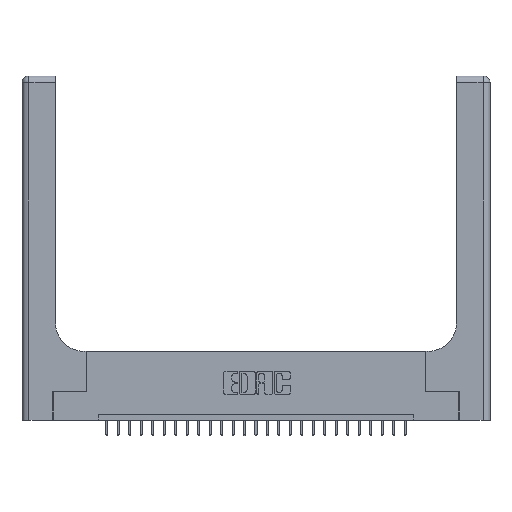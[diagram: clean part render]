
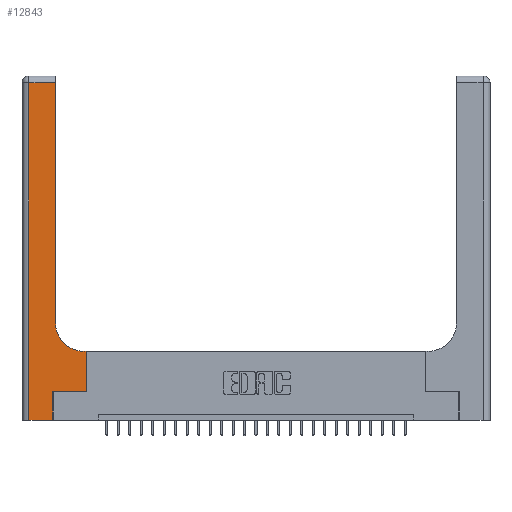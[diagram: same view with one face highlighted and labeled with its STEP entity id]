
A CAD part, top view. The second image highlights one B-rep face of the part: STEP entity #12843.
In plain terms, the highlighted planar face has unit normal (0, 0, 1).
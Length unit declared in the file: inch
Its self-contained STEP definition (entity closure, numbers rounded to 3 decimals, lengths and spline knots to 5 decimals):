
#403 = VERTEX_POINT ( 'NONE', #27520 ) ;
#743 = EDGE_LOOP ( 'NONE', ( #6027, #2777, #17085, #20887, #7346, #8097, #13744, #4555, #5136 ) ) ;
#778 = EDGE_CURVE ( 'NONE', #21902, #6032, #10229, .T. ) ;
#1618 = DIRECTION ( 'NONE',  ( 0., -1., 0. ) ) ;
#1889 = CARTESIAN_POINT ( 'NONE',  ( 0., 0., 0.37 ) ) ;
#2777 = ORIENTED_EDGE ( 'NONE', *, *, #16664, .T. ) ;
#3602 = CARTESIAN_POINT ( 'NONE',  ( 0.06, 2.94, 0.37 ) ) ;
#3624 = CARTESIAN_POINT ( 'NONE',  ( 0.269, 0., 0.37 ) ) ;
#4337 = DIRECTION ( 'NONE',  ( -1., 0., 0. ) ) ;
#4472 = CARTESIAN_POINT ( 'NONE',  ( 0.2915, 0.6, 0.37 ) ) ;
#4555 = ORIENTED_EDGE ( 'NONE', *, *, #15517, .T. ) ;
#5136 = ORIENTED_EDGE ( 'NONE', *, *, #16318, .T. ) ;
#5464 = DIRECTION ( 'NONE',  ( -1., 0., 0. ) ) ;
#5509 = LINE ( 'NONE', #5810, #17390 ) ;
#5621 = DIRECTION ( 'NONE',  ( -1., 0., 0. ) ) ;
#5810 = CARTESIAN_POINT ( 'NONE',  ( 0.06, 3., 0.37 ) ) ;
#6027 = ORIENTED_EDGE ( 'NONE', *, *, #16944, .T. ) ;
#6032 = VERTEX_POINT ( 'NONE', #25245 ) ;
#6249 = LINE ( 'NONE', #12702, #15602 ) ;
#6260 = EDGE_CURVE ( 'NONE', #12882, #21902, #9320, .T. ) ;
#6365 = DIRECTION ( 'NONE',  ( 1., 0., 0. ) ) ;
#6820 = LINE ( 'NONE', #4472, #7977 ) ;
#7346 = ORIENTED_EDGE ( 'NONE', *, *, #6260, .T. ) ;
#7562 = LINE ( 'NONE', #24616, #19625 ) ;
#7718 = CARTESIAN_POINT ( 'NONE',  ( 0., 3., 0.37 ) ) ;
#7977 = VECTOR ( 'NONE', #4337, 39.37008 ) ;
#8097 = ORIENTED_EDGE ( 'NONE', *, *, #778, .T. ) ;
#8233 = LINE ( 'NONE', #8536, #24083 ) ;
#8536 = CARTESIAN_POINT ( 'NONE',  ( 0.5585, 0.25, 0.37 ) ) ;
#9320 = LINE ( 'NONE', #19786, #27367 ) ;
#9348 = CIRCLE ( 'NONE', #10255, 0.25 ) ;
#9430 = FACE_OUTER_BOUND ( 'NONE', #743, .T. ) ;
#9842 = PLANE ( 'NONE',  #18192 ) ;
#10229 = LINE ( 'NONE', #16069, #27058 ) ;
#10255 = AXIS2_PLACEMENT_3D ( 'NONE', #17223, #19468, #25474 ) ;
#12702 = CARTESIAN_POINT ( 'NONE',  ( 0.2915, 3., 0.37 ) ) ;
#12843 = ADVANCED_FACE ( 'NONE', ( #9430 ), #9842, .F. ) ;
#12882 = VERTEX_POINT ( 'NONE', #3624 ) ;
#12930 = VERTEX_POINT ( 'NONE', #18705 ) ;
#13242 = VERTEX_POINT ( 'NONE', #24102 ) ;
#13744 = ORIENTED_EDGE ( 'NONE', *, *, #17756, .T. ) ;
#13872 = DIRECTION ( 'NONE',  ( 1., 0., 0. ) ) ;
#14234 = VERTEX_POINT ( 'NONE', #14402 ) ;
#14402 = CARTESIAN_POINT ( 'NONE',  ( 0.2915, 0.85, 0.37 ) ) ;
#15517 = EDGE_CURVE ( 'NONE', #403, #13242, #6820, .T. ) ;
#15602 = VECTOR ( 'NONE', #16732, 39.37008 ) ;
#16069 = CARTESIAN_POINT ( 'NONE',  ( 0.269, 0.25, 0.37 ) ) ;
#16318 = EDGE_CURVE ( 'NONE', #13242, #14234, #9348, .T. ) ;
#16664 = EDGE_CURVE ( 'NONE', #12930, #16796, #7562, .T. ) ;
#16732 = DIRECTION ( 'NONE',  ( 0., 1., 0. ) ) ;
#16796 = VERTEX_POINT ( 'NONE', #3602 ) ;
#16944 = EDGE_CURVE ( 'NONE', #14234, #12930, #6249, .T. ) ;
#17085 = ORIENTED_EDGE ( 'NONE', *, *, #23357, .T. ) ;
#17223 = CARTESIAN_POINT ( 'NONE',  ( 0.5415, 0.85, 0.37 ) ) ;
#17390 = VECTOR ( 'NONE', #1618, 39.37008 ) ;
#17756 = EDGE_CURVE ( 'NONE', #6032, #403, #8233, .T. ) ;
#18192 = AXIS2_PLACEMENT_3D ( 'NONE', #7718, #24766, #5621 ) ;
#18705 = CARTESIAN_POINT ( 'NONE',  ( 0.2915, 2.94, 0.37 ) ) ;
#19468 = DIRECTION ( 'NONE',  ( 0., 0., -1. ) ) ;
#19625 = VECTOR ( 'NONE', #5464, 39.37008 ) ;
#19786 = CARTESIAN_POINT ( 'NONE',  ( 0.269, 0., 0.37 ) ) ;
#20887 = ORIENTED_EDGE ( 'NONE', *, *, #25175, .T. ) ;
#21105 = DIRECTION ( 'NONE',  ( 0., 1., 0. ) ) ;
#21205 = CARTESIAN_POINT ( 'NONE',  ( 0.269, 0.25, 0.37 ) ) ;
#21902 = VERTEX_POINT ( 'NONE', #21205 ) ;
#21907 = VECTOR ( 'NONE', #6365, 39.37008 ) ;
#23235 = VERTEX_POINT ( 'NONE', #24364 ) ;
#23357 = EDGE_CURVE ( 'NONE', #16796, #23235, #5509, .T. ) ;
#24083 = VECTOR ( 'NONE', #21105, 39.37008 ) ;
#24102 = CARTESIAN_POINT ( 'NONE',  ( 0.5415, 0.6, 0.37 ) ) ;
#24364 = CARTESIAN_POINT ( 'NONE',  ( 0.06, 0., 0.37 ) ) ;
#24616 = CARTESIAN_POINT ( 'NONE',  ( 0., 2.94, 0.37 ) ) ;
#24766 = DIRECTION ( 'NONE',  ( 0., 0., -1. ) ) ;
#25175 = EDGE_CURVE ( 'NONE', #23235, #12882, #25489, .T. ) ;
#25245 = CARTESIAN_POINT ( 'NONE',  ( 0.5585, 0.25, 0.37 ) ) ;
#25474 = DIRECTION ( 'NONE',  ( 1., 0., 0. ) ) ;
#25489 = LINE ( 'NONE', #1889, #21907 ) ;
#26332 = DIRECTION ( 'NONE',  ( 0., 1., 0. ) ) ;
#27058 = VECTOR ( 'NONE', #13872, 39.37008 ) ;
#27367 = VECTOR ( 'NONE', #26332, 39.37008 ) ;
#27520 = CARTESIAN_POINT ( 'NONE',  ( 0.5585, 0.6, 0.37 ) ) ;
